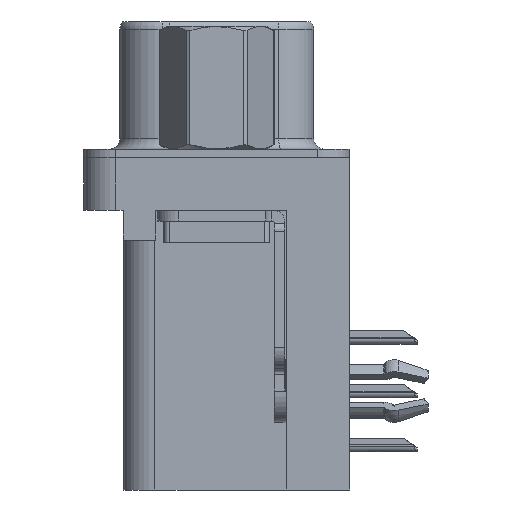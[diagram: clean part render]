
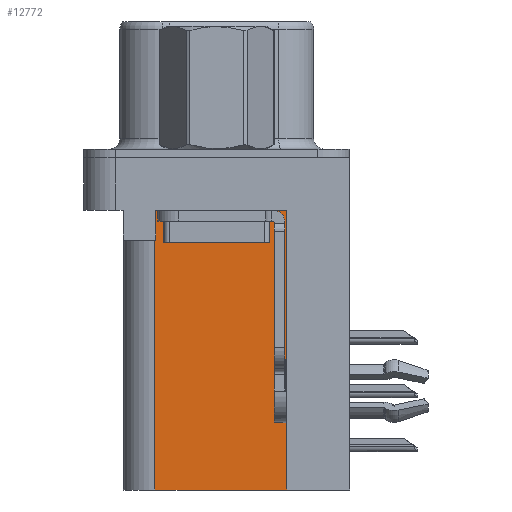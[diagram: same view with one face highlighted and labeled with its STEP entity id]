
A CAD part, left-side view. The second image highlights one B-rep face of the part: STEP entity #12772.
In plain terms, the highlighted planar face has unit normal (-1, 0, 0).
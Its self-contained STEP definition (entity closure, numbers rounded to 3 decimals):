
#60 = PLANE ( 'NONE',  #8332 ) ;
#419 = VERTEX_POINT ( 'NONE', #11264 ) ;
#958 = ORIENTED_EDGE ( 'NONE', *, *, #23676, .F. ) ;
#1230 = ORIENTED_EDGE ( 'NONE', *, *, #35344, .T. ) ;
#1735 = CARTESIAN_POINT ( 'NONE',  ( 3.7, 2.925, -15.7 ) ) ;
#2750 = CARTESIAN_POINT ( 'NONE',  ( 3.7, 2.895, -3.9 ) ) ;
#2901 = VECTOR ( 'NONE', #7140, 1000. ) ;
#2909 = CARTESIAN_POINT ( 'NONE',  ( 3.7, -3.295, -15.7 ) ) ;
#4357 = CARTESIAN_POINT ( 'NONE',  ( 3.7, 2.895, -3.9 ) ) ;
#6225 = VECTOR ( 'NONE', #13520, 1000. ) ;
#6762 = LINE ( 'NONE', #16307, #20536 ) ;
#7140 = DIRECTION ( 'NONE',  ( 0., 0., -1. ) ) ;
#8108 = VERTEX_POINT ( 'NONE', #22318 ) ;
#8332 = AXIS2_PLACEMENT_3D ( 'NONE', #2909, #11282, #30514 ) ;
#9495 = FACE_OUTER_BOUND ( 'NONE', #20581, .T. ) ;
#10451 = VECTOR ( 'NONE', #33431, 1000. ) ;
#11264 = CARTESIAN_POINT ( 'NONE',  ( 3.7, 2.895, -2.5 ) ) ;
#11282 = DIRECTION ( 'NONE',  ( 1., 0., 0. ) ) ;
#11320 = LINE ( 'NONE', #30589, #10451 ) ;
#11555 = LINE ( 'NONE', #27722, #17968 ) ;
#11896 = EDGE_CURVE ( 'NONE', #23423, #419, #15306, .T. ) ;
#12772 = ADVANCED_FACE ( 'NONE', ( #9495 ), #60, .F. ) ;
#13520 = DIRECTION ( 'NONE',  ( 0., 1., 0. ) ) ;
#13584 = LINE ( 'NONE', #18881, #6225 ) ;
#14124 = VERTEX_POINT ( 'NONE', #1735 ) ;
#14221 = ORIENTED_EDGE ( 'NONE', *, *, #11896, .T. ) ;
#15306 = LINE ( 'NONE', #16148, #29916 ) ;
#15426 = VERTEX_POINT ( 'NONE', #2750 ) ;
#16148 = CARTESIAN_POINT ( 'NONE',  ( 3.7, -3.295, -2.5 ) ) ;
#16307 = CARTESIAN_POINT ( 'NONE',  ( 3.7, -3.295, -15.7 ) ) ;
#17581 = LINE ( 'NONE', #4357, #2901 ) ;
#17968 = VECTOR ( 'NONE', #24973, 1000. ) ;
#18052 = ORIENTED_EDGE ( 'NONE', *, *, #34075, .T. ) ;
#18881 = CARTESIAN_POINT ( 'NONE',  ( 3.7, 0., -3.9 ) ) ;
#20536 = VECTOR ( 'NONE', #35677, 1000. ) ;
#20581 = EDGE_LOOP ( 'NONE', ( #14221, #22702, #18052, #958, #29346, #1230 ) ) ;
#22005 = VERTEX_POINT ( 'NONE', #26955 ) ;
#22318 = CARTESIAN_POINT ( 'NONE',  ( 3.7, 2.925, -3.9 ) ) ;
#22702 = ORIENTED_EDGE ( 'NONE', *, *, #30542, .T. ) ;
#23423 = VERTEX_POINT ( 'NONE', #35101 ) ;
#23676 = EDGE_CURVE ( 'NONE', #14124, #8108, #11555, .T. ) ;
#24973 = DIRECTION ( 'NONE',  ( 0., 0., 1. ) ) ;
#26955 = CARTESIAN_POINT ( 'NONE',  ( 3.7, -3.295, -15.7 ) ) ;
#27722 = CARTESIAN_POINT ( 'NONE',  ( 3.7, 2.925, -15.7 ) ) ;
#27813 = EDGE_CURVE ( 'NONE', #22005, #14124, #11320, .T. ) ;
#29346 = ORIENTED_EDGE ( 'NONE', *, *, #27813, .F. ) ;
#29916 = VECTOR ( 'NONE', #35524, 1000. ) ;
#30514 = DIRECTION ( 'NONE',  ( 0., 0., -1. ) ) ;
#30542 = EDGE_CURVE ( 'NONE', #419, #15426, #17581, .T. ) ;
#30589 = CARTESIAN_POINT ( 'NONE',  ( 3.7, -3.295, -15.7 ) ) ;
#33431 = DIRECTION ( 'NONE',  ( 0., 1., 0. ) ) ;
#34075 = EDGE_CURVE ( 'NONE', #15426, #8108, #13584, .T. ) ;
#35101 = CARTESIAN_POINT ( 'NONE',  ( 3.7, -3.295, -2.5 ) ) ;
#35344 = EDGE_CURVE ( 'NONE', #22005, #23423, #6762, .T. ) ;
#35524 = DIRECTION ( 'NONE',  ( 0., 1., 0. ) ) ;
#35677 = DIRECTION ( 'NONE',  ( 0., 0., 1. ) ) ;
